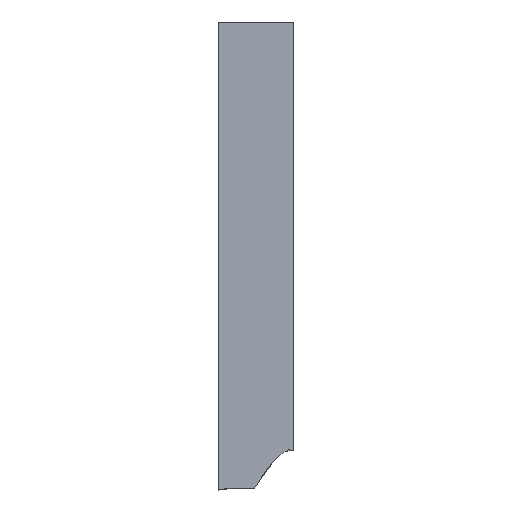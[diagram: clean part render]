
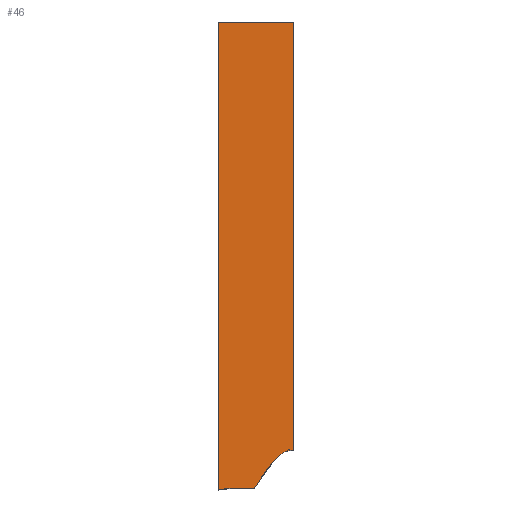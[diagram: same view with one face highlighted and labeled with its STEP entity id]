
A CAD part, top view. The second image highlights one B-rep face of the part: STEP entity #46.
In plain terms, the highlighted planar face has unit normal (0, 0, 1).
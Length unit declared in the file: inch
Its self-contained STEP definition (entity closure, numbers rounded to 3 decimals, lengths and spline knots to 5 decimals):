
#30 = DIRECTION ( 'NONE',  ( 0., 1., 0. ) ) ;
#43 = PLANE ( 'NONE',  #290 ) ;
#46 = ADVANCED_FACE ( 'NONE', ( #1075 ), #43, .T. ) ;
#74 = DIRECTION ( 'NONE',  ( 0., 1., 0. ) ) ;
#85 = VERTEX_POINT ( 'NONE', #1361 ) ;
#98 = VECTOR ( 'NONE', #1469, 39.37008 ) ;
#107 = ORIENTED_EDGE ( 'NONE', *, *, #243, .T. ) ;
#108 = CARTESIAN_POINT ( 'NONE',  ( -0.2782, -1.9735, 0.4665 ) ) ;
#116 = EDGE_CURVE ( 'NONE', #707, #1069, #756, .T. ) ;
#123 = LINE ( 'NONE', #1048, #826 ) ;
#170 = AXIS2_PLACEMENT_3D ( 'NONE', #1524, #734, #1652 ) ;
#203 = CARTESIAN_POINT ( 'NONE',  ( -1.02672, -2.07217, 0.4665 ) ) ;
#243 = EDGE_CURVE ( 'NONE', #295, #85, #1381, .T. ) ;
#262 = CARTESIAN_POINT ( 'NONE',  ( -0.25412, -1.94265, 0.4665 ) ) ;
#290 = AXIS2_PLACEMENT_3D ( 'NONE', #203, #1671, #1281 ) ;
#295 = VERTEX_POINT ( 'NONE', #880 ) ;
#309 = CARTESIAN_POINT ( 'NONE',  ( -0.15996, -1.88797, 0.4665 ) ) ;
#322 = VECTOR ( 'NONE', #30, 39.37008 ) ;
#372 = VERTEX_POINT ( 'NONE', #1129 ) ;
#396 = CARTESIAN_POINT ( 'NONE',  ( -0.33314, -2.0545, 0.4665 ) ) ;
#400 = CARTESIAN_POINT ( 'NONE',  ( -0.23465, -1.9207, 0.4665 ) ) ;
#402 = EDGE_CURVE ( 'NONE', #295, #707, #777, .T. ) ;
#525 = EDGE_CURVE ( 'NONE', #372, #85, #1325, .T. ) ;
#535 = CARTESIAN_POINT ( 'NONE',  ( -0.1762, -1.88797, 0.4665 ) ) ;
#546 = CARTESIAN_POINT ( 'NONE',  ( -0.21283, -1.90115, 0.4665 ) ) ;
#555 = CARTESIAN_POINT ( 'NONE',  ( -0.1762, -1.88797, 0.4665 ) ) ;
#598 = EDGE_CURVE ( 'NONE', #372, #1081, #1565, .T. ) ;
#605 = EDGE_CURVE ( 'NONE', #1081, #721, #1581, .T. ) ;
#673 = CARTESIAN_POINT ( 'NONE',  ( -0.19553, -1.89173, 0.4665 ) ) ;
#686 = CARTESIAN_POINT ( 'NONE',  ( 2.5093, 0., 0.4665 ) ) ;
#707 = VERTEX_POINT ( 'NONE', #991 ) ;
#721 = VERTEX_POINT ( 'NONE', #309 ) ;
#727 = ORIENTED_EDGE ( 'NONE', *, *, #402, .F. ) ;
#734 = DIRECTION ( 'NONE',  ( 0., 0., -1. ) ) ;
#747 = ORIENTED_EDGE ( 'NONE', *, *, #598, .T. ) ;
#756 = LINE ( 'NONE', #686, #1029 ) ;
#775 = EDGE_CURVE ( 'NONE', #721, #1069, #123, .T. ) ;
#777 = LINE ( 'NONE', #875, #322 ) ;
#808 = CARTESIAN_POINT ( 'NONE',  ( -0.32249, -2.03808, 0.4665 ) ) ;
#816 = CARTESIAN_POINT ( 'NONE',  ( -0.18118, -1.88797, 0.4665 ) ) ;
#826 = VECTOR ( 'NONE', #74, 39.37008 ) ;
#875 = CARTESIAN_POINT ( 'NONE',  ( -0.49053, -0.335, 0.4665 ) ) ;
#880 = CARTESIAN_POINT ( 'NONE',  ( -0.49053, -2.06046, 0.4665 ) ) ;
#944 = CARTESIAN_POINT ( 'NONE',  ( -0.28955, -1.98947, 0.4665 ) ) ;
#954 = EDGE_LOOP ( 'NONE', ( #1260, #1146, #1448, #727, #107, #1043, #747 ) ) ;
#973 = VECTOR ( 'NONE', #1328, 39.37008 ) ;
#991 = CARTESIAN_POINT ( 'NONE',  ( -0.49053, 0., 0.4665 ) ) ;
#1029 = VECTOR ( 'NONE', #1220, 39.37008 ) ;
#1043 = ORIENTED_EDGE ( 'NONE', *, *, #525, .F. ) ;
#1048 = CARTESIAN_POINT ( 'NONE',  ( -0.15996, 0., 0.4665 ) ) ;
#1069 = VERTEX_POINT ( 'NONE', #1459 ) ;
#1075 = FACE_OUTER_BOUND ( 'NONE', #954, .T. ) ;
#1081 = VERTEX_POINT ( 'NONE', #535 ) ;
#1082 = CARTESIAN_POINT ( 'NONE',  ( -0.26026, -1.95027, 0.4665 ) ) ;
#1129 = CARTESIAN_POINT ( 'NONE',  ( -0.33314, -2.0545, 0.4665 ) ) ;
#1146 = ORIENTED_EDGE ( 'NONE', *, *, #775, .T. ) ;
#1204 = CARTESIAN_POINT ( 'NONE',  ( -0.24129, -1.92785, 0.4665 ) ) ;
#1220 = DIRECTION ( 'NONE',  ( 1., 0., 0. ) ) ;
#1260 = ORIENTED_EDGE ( 'NONE', *, *, #605, .T. ) ;
#1281 = DIRECTION ( 'NONE',  ( 1., 0., 0. ) ) ;
#1325 = LINE ( 'NONE', #1576, #973 ) ;
#1328 = DIRECTION ( 'NONE',  ( -1., 0., 0. ) ) ;
#1344 = CARTESIAN_POINT ( 'NONE',  ( -0.22044, -1.9074, 0.4665 ) ) ;
#1361 = CARTESIAN_POINT ( 'NONE',  ( -0.41423, -2.0545, 0.4665 ) ) ;
#1381 = CIRCLE ( 'NONE', #170, 0.49213 ) ;
#1448 = ORIENTED_EDGE ( 'NONE', *, *, #116, .F. ) ;
#1459 = CARTESIAN_POINT ( 'NONE',  ( -0.15996, 0., 0.4665 ) ) ;
#1463 = CARTESIAN_POINT ( 'NONE',  ( -0.19999, -1.89379, 0.4665 ) ) ;
#1469 = DIRECTION ( 'NONE',  ( 1., 0., 0. ) ) ;
#1524 = CARTESIAN_POINT ( 'NONE',  ( -0.41423, -2.54663, 0.4665 ) ) ;
#1565 = B_SPLINE_CURVE_WITH_KNOTS ( 'NONE', 3,
 ( #396, #808, #1731, #944, #108, #1082, #262, #1204, #400, #1344, #546, #1463, #673, #1596, #816, #1735 ),
 .UNSPECIFIED., .F., .F.,
 ( 4, 2, 2, 2, 2, 2, 2, 4 ),
 ( 0., 0.00149, 0.00298, 0.00373, 0.00447, 0.00522, 0.00559, 0.00597 ),
 .UNSPECIFIED. ) ;
#1576 = CARTESIAN_POINT ( 'NONE',  ( 0., -2.0545, 0.4665 ) ) ;
#1581 = LINE ( 'NONE', #555, #98 ) ;
#1596 = CARTESIAN_POINT ( 'NONE',  ( -0.18608, -1.88879, 0.4665 ) ) ;
#1652 = DIRECTION ( 'NONE',  ( 1., 0., 0. ) ) ;
#1671 = DIRECTION ( 'NONE',  ( 0., 0., 1. ) ) ;
#1731 = CARTESIAN_POINT ( 'NONE',  ( -0.3117, -2.02175, 0.4665 ) ) ;
#1735 = CARTESIAN_POINT ( 'NONE',  ( -0.1762, -1.88797, 0.4665 ) ) ;
